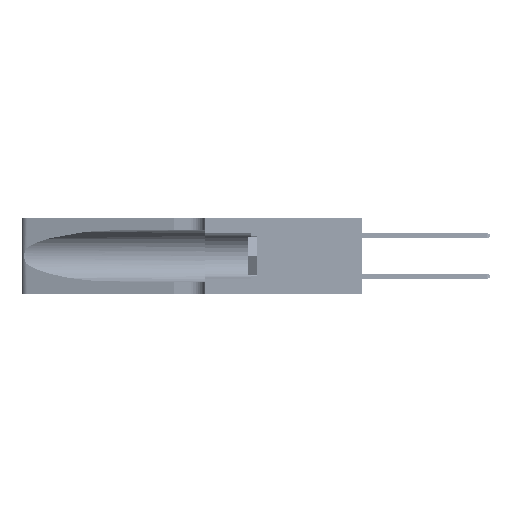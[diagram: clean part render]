
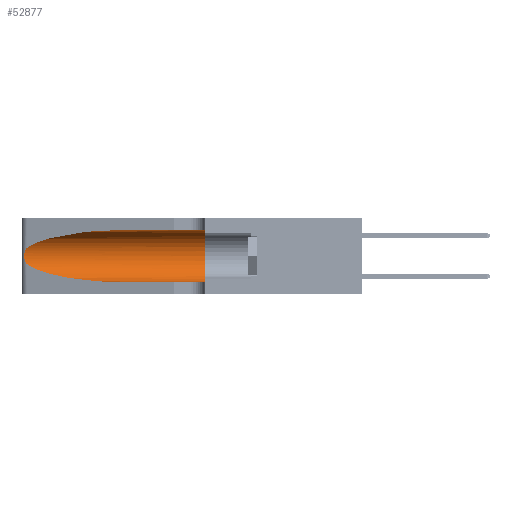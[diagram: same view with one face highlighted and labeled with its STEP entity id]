
A CAD part, left-side view. The second image highlights one B-rep face of the part: STEP entity #52877.
In plain terms, the highlighted cylindrical face has radius 3.308 mm (diameter 6.617 mm), a partial arc.
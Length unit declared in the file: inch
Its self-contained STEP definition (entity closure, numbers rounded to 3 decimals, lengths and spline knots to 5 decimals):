
#2106 = CARTESIAN_POINT ( 'NONE',  ( 0.25487, 1.22718, 0.14631 ) ) ;
#2242 = CARTESIAN_POINT ( 'NONE',  ( 0.25487, 1.22718, 0.14631 ) ) ;
#2290 = CARTESIAN_POINT ( 'NONE',  ( 0.25639, 1.23184, 0.21858 ) ) ;
#3336 = EDGE_CURVE ( 'NONE', #44087, #10149, #9003, .T. ) ;
#4248 = DIRECTION ( 'NONE',  ( 0., 0., -1. ) ) ;
#5350 = VERTEX_POINT ( 'NONE', #50529 ) ;
#6754 = VERTEX_POINT ( 'NONE', #43250 ) ;
#7643 = EDGE_CURVE ( 'NONE', #6754, #8766, #33971, .T. ) ;
#8174 = VECTOR ( 'NONE', #14676, 39.37008 ) ;
#8689 = CARTESIAN_POINT ( 'NONE',  ( 0.25487, 1.22718, 0.22369 ) ) ;
#8766 = VERTEX_POINT ( 'NONE', #41626 ) ;
#9003 = CIRCLE ( 'NONE', #13155, 0.13025 ) ;
#9525 = ORIENTED_EDGE ( 'NONE', *, *, #17502, .T. ) ;
#10149 = VERTEX_POINT ( 'NONE', #17202 ) ;
#10193 = CARTESIAN_POINT ( 'NONE',  ( 0.1305, 0.35, 0.31525 ) ) ;
#10341 = CARTESIAN_POINT ( 'NONE',  ( 0.25789, 1.23486, 0.15765 ) ) ;
#11270 = EDGE_CURVE ( 'NONE', #18764, #10149, #46453, .T. ) ;
#11351 = ORIENTED_EDGE ( 'NONE', *, *, #41569, .F. ) ;
#13155 = AXIS2_PLACEMENT_3D ( 'NONE', #30627, #22210, #51490 ) ;
#14486 = B_SPLINE_CURVE_WITH_KNOTS ( 'NONE', 3,
 ( #43408, #18379, #2290, #47807, #22761, #18564, #35924, #18927, #35389, #27687, #10341, #47983, #27328, #2106 ),
 .UNSPECIFIED., .F., .F.,
 ( 4, 2, 2, 2, 2, 2, 4 ),
 ( 0., 0.00027, 0.00053, 0.00107, 0.0016, 0.00187, 0.00214 ),
 .UNSPECIFIED. ) ;
#14676 = DIRECTION ( 'NONE',  ( 0., -1., 0. ) ) ;
#16909 = CARTESIAN_POINT ( 'NONE',  ( 0.1305, 1.61858, 0.05475 ) ) ;
#17202 = CARTESIAN_POINT ( 'NONE',  ( 0.1305, 0.35, 0.05475 ) ) ;
#17502 = EDGE_CURVE ( 'NONE', #8766, #5350, #14486, .T. ) ;
#18379 = CARTESIAN_POINT ( 'NONE',  ( 0.25555, 1.22994, 0.2215 ) ) ;
#18564 = CARTESIAN_POINT ( 'NONE',  ( 0.26018, 1.23835, 0.19895 ) ) ;
#18764 = VERTEX_POINT ( 'NONE', #21920 ) ;
#18927 = CARTESIAN_POINT ( 'NONE',  ( 0.26075, 1.23896, 0.178 ) ) ;
#19330 = LINE ( 'NONE', #39752, #8174 ) ;
#19674 = VECTOR ( 'NONE', #28984, 39.37008 ) ;
#20528 = EDGE_CURVE ( 'NONE', #5350, #18764, #21183, .T. ) ;
#20531 = AXIS2_PLACEMENT_3D ( 'NONE', #53948, #41319, #4248 ) ;
#21183 =( BOUNDED_CURVE ( )  B_SPLINE_CURVE ( 3, ( #2242, #39503, #52500, #27459 ),
 .UNSPECIFIED., .F., .T. ) 
 B_SPLINE_CURVE_WITH_KNOTS ( ( 4, 4 ),
 ( 3.44316, 4.71239 ),
 .UNSPECIFIED. ) 
 CURVE ( )  GEOMETRIC_REPRESENTATION_ITEM ( )  RATIONAL_B_SPLINE_CURVE ( ( 1., 0.87, 0.87, 1. ) ) 
 REPRESENTATION_ITEM ( '' )  );
#21920 = CARTESIAN_POINT ( 'NONE',  ( 0.1305, 0.72297, 0.05475 ) ) ;
#22046 = CARTESIAN_POINT ( 'NONE',  ( 0.1305, 0.72297, 0.31525 ) ) ;
#22210 = DIRECTION ( 'NONE',  ( 0., 1., 0. ) ) ;
#22761 = CARTESIAN_POINT ( 'NONE',  ( 0.25854, 1.2359, 0.20912 ) ) ;
#25462 = ORIENTED_EDGE ( 'NONE', *, *, #11270, .T. ) ;
#26672 = EDGE_LOOP ( 'NONE', ( #44733, #9525, #28553, #25462, #48097, #11351 ) ) ;
#27328 = CARTESIAN_POINT ( 'NONE',  ( 0.25555, 1.22993, 0.14849 ) ) ;
#27459 = CARTESIAN_POINT ( 'NONE',  ( 0.1305, 0.72297, 0.05475 ) ) ;
#27687 = CARTESIAN_POINT ( 'NONE',  ( 0.25856, 1.23593, 0.16098 ) ) ;
#28553 = ORIENTED_EDGE ( 'NONE', *, *, #20528, .T. ) ;
#28688 = CYLINDRICAL_SURFACE ( 'NONE', #20531, 0.13025 ) ;
#28984 = DIRECTION ( 'NONE',  ( 0., -1., 0. ) ) ;
#30078 = CARTESIAN_POINT ( 'NONE',  ( 0.18966, 0.96281, 0.31525 ) ) ;
#30627 = CARTESIAN_POINT ( 'NONE',  ( 0.1305, 0.35, 0.185 ) ) ;
#33761 = CARTESIAN_POINT ( 'NONE',  ( 0.2373, 1.15595, 0.28018 ) ) ;
#33971 =( BOUNDED_CURVE ( )  B_SPLINE_CURVE ( 3, ( #22046, #30078, #33761, #8689 ),
 .UNSPECIFIED., .F., .F. ) 
 B_SPLINE_CURVE_WITH_KNOTS ( ( 4, 4 ),
 ( 1.5708, 2.84003 ),
 .UNSPECIFIED. ) 
 CURVE ( )  GEOMETRIC_REPRESENTATION_ITEM ( )  RATIONAL_B_SPLINE_CURVE ( ( 1., 0.87, 0.87, 1. ) ) 
 REPRESENTATION_ITEM ( '' )  );
#35389 = CARTESIAN_POINT ( 'NONE',  ( 0.26017, 1.23833, 0.17102 ) ) ;
#35924 = CARTESIAN_POINT ( 'NONE',  ( 0.26075, 1.23896, 0.19203 ) ) ;
#37816 = FACE_OUTER_BOUND ( 'NONE', #26672, .T. ) ;
#39503 = CARTESIAN_POINT ( 'NONE',  ( 0.2373, 1.15595, 0.08982 ) ) ;
#39752 = CARTESIAN_POINT ( 'NONE',  ( 0.1305, 1.61858, 0.31525 ) ) ;
#41319 = DIRECTION ( 'NONE',  ( 0., -1., 0. ) ) ;
#41569 = EDGE_CURVE ( 'NONE', #6754, #44087, #19330, .T. ) ;
#41626 = CARTESIAN_POINT ( 'NONE',  ( 0.25487, 1.22718, 0.22369 ) ) ;
#43250 = CARTESIAN_POINT ( 'NONE',  ( 0.1305, 0.72297, 0.31525 ) ) ;
#43408 = CARTESIAN_POINT ( 'NONE',  ( 0.25487, 1.22718, 0.22369 ) ) ;
#44087 = VERTEX_POINT ( 'NONE', #10193 ) ;
#44733 = ORIENTED_EDGE ( 'NONE', *, *, #7643, .T. ) ;
#46453 = LINE ( 'NONE', #16909, #19674 ) ;
#47807 = CARTESIAN_POINT ( 'NONE',  ( 0.25787, 1.23484, 0.2124 ) ) ;
#47983 = CARTESIAN_POINT ( 'NONE',  ( 0.25639, 1.23186, 0.15144 ) ) ;
#48097 = ORIENTED_EDGE ( 'NONE', *, *, #3336, .F. ) ;
#50529 = CARTESIAN_POINT ( 'NONE',  ( 0.25487, 1.22718, 0.14631 ) ) ;
#51490 = DIRECTION ( 'NONE',  ( 0., 0., 1. ) ) ;
#52500 = CARTESIAN_POINT ( 'NONE',  ( 0.18966, 0.96281, 0.05475 ) ) ;
#52877 = ADVANCED_FACE ( 'NONE', ( #37816 ), #28688, .F. ) ;
#53948 = CARTESIAN_POINT ( 'NONE',  ( 0.1305, 1.61858, 0.185 ) ) ;
